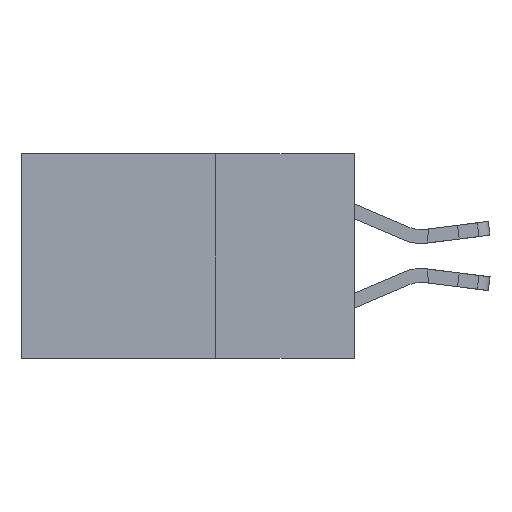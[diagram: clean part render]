
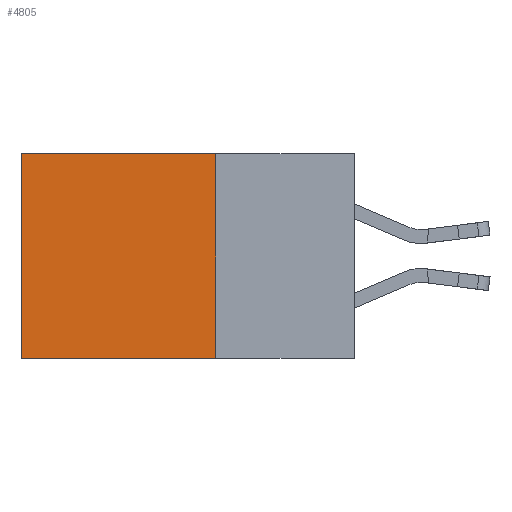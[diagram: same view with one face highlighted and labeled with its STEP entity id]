
A CAD part, left-side view. The second image highlights one B-rep face of the part: STEP entity #4805.
In plain terms, the highlighted planar face has unit normal (-1, 0, 0).
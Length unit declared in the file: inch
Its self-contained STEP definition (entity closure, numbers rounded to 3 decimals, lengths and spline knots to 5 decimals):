
#1359 = EDGE_LOOP ( 'NONE', ( #12426, #12838, #9494, #13330 ) ) ;
#1852 = CARTESIAN_POINT ( 'NONE',  ( 0.2615, 0.6, 0. ) ) ;
#3078 = CARTESIAN_POINT ( 'NONE',  ( 0.2615, 0.6, -0.37 ) ) ;
#4221 = EDGE_CURVE ( 'NONE', #4835, #6663, #8539, .T. ) ;
#4805 = ADVANCED_FACE ( 'NONE', ( #13563 ), #15903, .F. ) ;
#4835 = VERTEX_POINT ( 'NONE', #8993 ) ;
#5828 = VECTOR ( 'NONE', #11777, 39.37008 ) ;
#6137 = CARTESIAN_POINT ( 'NONE',  ( 0.2615, 0.6, -0.37 ) ) ;
#6151 = LINE ( 'NONE', #13840, #12642 ) ;
#6663 = VERTEX_POINT ( 'NONE', #1852 ) ;
#7408 = DIRECTION ( 'NONE',  ( 0., 0., -1. ) ) ;
#8304 = DIRECTION ( 'NONE',  ( 0., 0., -1. ) ) ;
#8539 = LINE ( 'NONE', #15498, #11612 ) ;
#8993 = CARTESIAN_POINT ( 'NONE',  ( 0.2615, 0.25, 0. ) ) ;
#9494 = ORIENTED_EDGE ( 'NONE', *, *, #12424, .F. ) ;
#9930 = VERTEX_POINT ( 'NONE', #16300 ) ;
#10517 = CARTESIAN_POINT ( 'NONE',  ( 0.2615, 0.25, -0.37 ) ) ;
#10882 = VECTOR ( 'NONE', #14649, 39.37008 ) ;
#11612 = VECTOR ( 'NONE', #15060, 39.37008 ) ;
#11777 = DIRECTION ( 'NONE',  ( 0., 1., 0. ) ) ;
#12424 = EDGE_CURVE ( 'NONE', #4835, #9930, #6151, .T. ) ;
#12426 = ORIENTED_EDGE ( 'NONE', *, *, #13512, .T. ) ;
#12642 = VECTOR ( 'NONE', #7408, 39.37008 ) ;
#12838 = ORIENTED_EDGE ( 'NONE', *, *, #16526, .F. ) ;
#13112 = LINE ( 'NONE', #10517, #5828 ) ;
#13330 = ORIENTED_EDGE ( 'NONE', *, *, #4221, .T. ) ;
#13512 = EDGE_CURVE ( 'NONE', #6663, #15686, #14895, .T. ) ;
#13563 = FACE_OUTER_BOUND ( 'NONE', #1359, .T. ) ;
#13840 = CARTESIAN_POINT ( 'NONE',  ( 0.2615, 0.25, -0.37 ) ) ;
#13942 = AXIS2_PLACEMENT_3D ( 'NONE', #14812, #15930, #8304 ) ;
#14649 = DIRECTION ( 'NONE',  ( 0., 0., -1. ) ) ;
#14812 = CARTESIAN_POINT ( 'NONE',  ( 0.2615, 0.25, -0.37 ) ) ;
#14895 = LINE ( 'NONE', #3078, #10882 ) ;
#15060 = DIRECTION ( 'NONE',  ( 0., 1., 0. ) ) ;
#15498 = CARTESIAN_POINT ( 'NONE',  ( 0.2615, 0.25, 0. ) ) ;
#15686 = VERTEX_POINT ( 'NONE', #6137 ) ;
#15903 = PLANE ( 'NONE',  #13942 ) ;
#15930 = DIRECTION ( 'NONE',  ( 1., 0., 0. ) ) ;
#16300 = CARTESIAN_POINT ( 'NONE',  ( 0.2615, 0.25, -0.37 ) ) ;
#16526 = EDGE_CURVE ( 'NONE', #9930, #15686, #13112, .T. ) ;
